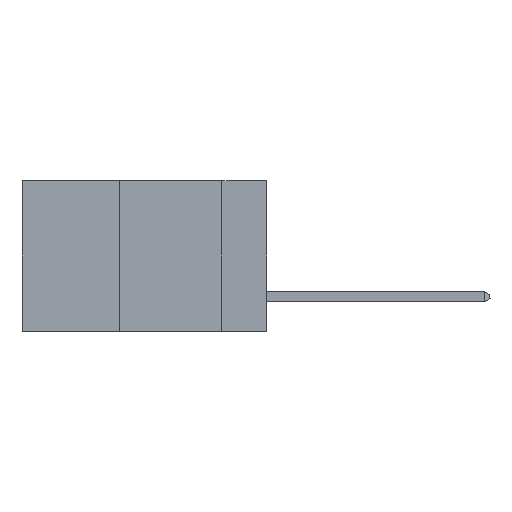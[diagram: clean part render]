
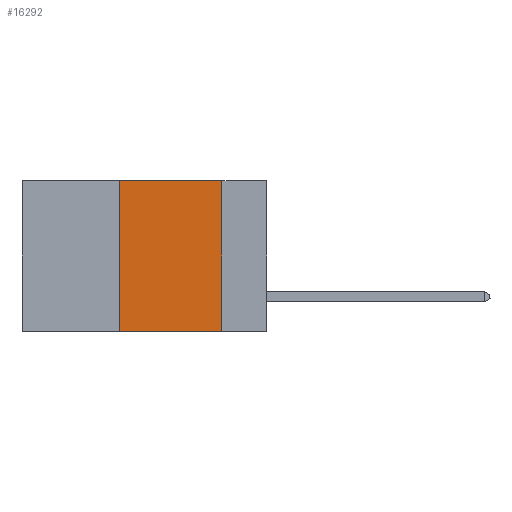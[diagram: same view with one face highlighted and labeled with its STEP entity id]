
A CAD part, left-side view. The second image highlights one B-rep face of the part: STEP entity #16292.
In plain terms, the highlighted planar face has unit normal (-1, 0, 0).
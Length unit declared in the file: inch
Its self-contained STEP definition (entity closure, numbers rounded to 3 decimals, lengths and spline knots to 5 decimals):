
#120 = CARTESIAN_POINT ( 'NONE',  ( 0., 0.11, 0. ) ) ;
#322 = CARTESIAN_POINT ( 'NONE',  ( 0., 0.36, 0. ) ) ;
#1062 = CARTESIAN_POINT ( 'NONE',  ( 0., 0.11, 0. ) ) ;
#1942 = CARTESIAN_POINT ( 'NONE',  ( 0., 0.36, 0. ) ) ;
#3463 = CARTESIAN_POINT ( 'NONE',  ( 0., 0.6, 0. ) ) ;
#4078 = VERTEX_POINT ( 'NONE', #14301 ) ;
#4399 = EDGE_CURVE ( 'NONE', #4078, #11880, #4918, .T. ) ;
#4576 = AXIS2_PLACEMENT_3D ( 'NONE', #3463, #9311, #15053 ) ;
#4886 = FACE_OUTER_BOUND ( 'NONE', #14745, .T. ) ;
#4918 = LINE ( 'NONE', #9016, #7877 ) ;
#4968 = LINE ( 'NONE', #7839, #8372 ) ;
#5009 = ORIENTED_EDGE ( 'NONE', *, *, #14225, .F. ) ;
#5010 = DIRECTION ( 'NONE',  ( 0., 0., 1. ) ) ;
#6509 = VECTOR ( 'NONE', #5010, 39.37008 ) ;
#7839 = CARTESIAN_POINT ( 'NONE',  ( 0., 0.6, 0. ) ) ;
#7877 = VECTOR ( 'NONE', #13460, 39.37008 ) ;
#8372 = VECTOR ( 'NONE', #9426, 39.37008 ) ;
#8597 = DIRECTION ( 'NONE',  ( 0., 0., -1. ) ) ;
#8812 = ORIENTED_EDGE ( 'NONE', *, *, #13833, .F. ) ;
#8822 = VECTOR ( 'NONE', #8597, 39.37008 ) ;
#9016 = CARTESIAN_POINT ( 'NONE',  ( 0., 0.6, -0.37 ) ) ;
#9311 = DIRECTION ( 'NONE',  ( 1., 0., 0. ) ) ;
#9426 = DIRECTION ( 'NONE',  ( 0., -1., 0. ) ) ;
#9502 = EDGE_CURVE ( 'NONE', #4078, #12199, #15383, .T. ) ;
#11880 = VERTEX_POINT ( 'NONE', #13410 ) ;
#12039 = PLANE ( 'NONE',  #4576 ) ;
#12199 = VERTEX_POINT ( 'NONE', #322 ) ;
#12684 = LINE ( 'NONE', #120, #8822 ) ;
#13410 = CARTESIAN_POINT ( 'NONE',  ( 0., 0.11, -0.37 ) ) ;
#13460 = DIRECTION ( 'NONE',  ( 0., -1., 0. ) ) ;
#13833 = EDGE_CURVE ( 'NONE', #12199, #16050, #4968, .T. ) ;
#13982 = ORIENTED_EDGE ( 'NONE', *, *, #9502, .F. ) ;
#14225 = EDGE_CURVE ( 'NONE', #16050, #11880, #12684, .T. ) ;
#14301 = CARTESIAN_POINT ( 'NONE',  ( 0., 0.36, -0.37 ) ) ;
#14745 = EDGE_LOOP ( 'NONE', ( #5009, #8812, #13982, #16886 ) ) ;
#15053 = DIRECTION ( 'NONE',  ( 0., 0., -1. ) ) ;
#15383 = LINE ( 'NONE', #1942, #6509 ) ;
#16050 = VERTEX_POINT ( 'NONE', #1062 ) ;
#16292 = ADVANCED_FACE ( 'NONE', ( #4886 ), #12039, .F. ) ;
#16886 = ORIENTED_EDGE ( 'NONE', *, *, #4399, .T. ) ;
